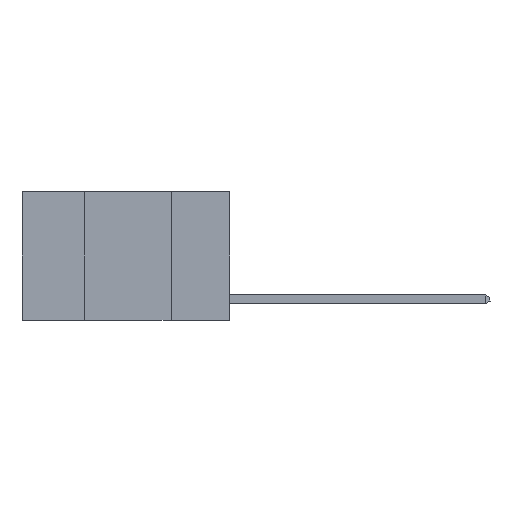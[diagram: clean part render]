
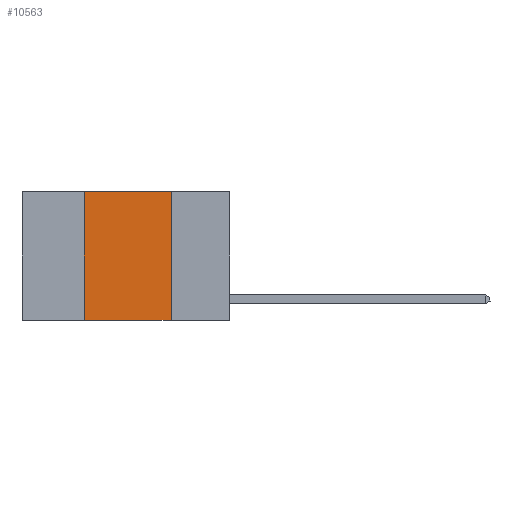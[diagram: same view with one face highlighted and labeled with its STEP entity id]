
A CAD part, left-side view. The second image highlights one B-rep face of the part: STEP entity #10563.
In plain terms, the highlighted planar face has unit normal (-1, 0, 0).
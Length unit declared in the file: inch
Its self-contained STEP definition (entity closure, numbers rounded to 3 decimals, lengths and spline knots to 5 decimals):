
#159 = ORIENTED_EDGE ( 'NONE', *, *, #10945, .T. ) ;
#647 = EDGE_CURVE ( 'NONE', #4507, #5909, #17283, .T. ) ;
#2080 = CARTESIAN_POINT ( 'NONE',  ( 0., 0.42, 0. ) ) ;
#2195 = CARTESIAN_POINT ( 'NONE',  ( 0., 0.6, -0.37 ) ) ;
#2714 = VECTOR ( 'NONE', #12635, 39.37008 ) ;
#2931 = CARTESIAN_POINT ( 'NONE',  ( 0., 0.42, 0. ) ) ;
#3267 = LINE ( 'NONE', #2195, #2714 ) ;
#3363 = CARTESIAN_POINT ( 'NONE',  ( 0., 0.42, -0.37 ) ) ;
#3671 = ORIENTED_EDGE ( 'NONE', *, *, #13306, .F. ) ;
#3960 = CARTESIAN_POINT ( 'NONE',  ( 0., 0.17, 0. ) ) ;
#4500 = VECTOR ( 'NONE', #12670, 39.37008 ) ;
#4507 = VERTEX_POINT ( 'NONE', #2931 ) ;
#5380 = VECTOR ( 'NONE', #19575, 39.37008 ) ;
#5909 = VERTEX_POINT ( 'NONE', #13695 ) ;
#7539 = CARTESIAN_POINT ( 'NONE',  ( 0., 0.6, 0. ) ) ;
#7980 = VECTOR ( 'NONE', #16183, 39.37008 ) ;
#9848 = CARTESIAN_POINT ( 'NONE',  ( 0., 0.6, 0. ) ) ;
#9978 = LINE ( 'NONE', #2080, #5380 ) ;
#10563 = ADVANCED_FACE ( 'NONE', ( #15002 ), #20243, .F. ) ;
#10945 = EDGE_CURVE ( 'NONE', #13084, #15757, #3267, .T. ) ;
#11211 = EDGE_LOOP ( 'NONE', ( #3671, #12945, #17567, #159 ) ) ;
#11629 = DIRECTION ( 'NONE',  ( 0., 0., -1. ) ) ;
#12132 = EDGE_CURVE ( 'NONE', #13084, #4507, #9978, .T. ) ;
#12635 = DIRECTION ( 'NONE',  ( 0., -1., 0. ) ) ;
#12670 = DIRECTION ( 'NONE',  ( 0., 0., -1. ) ) ;
#12945 = ORIENTED_EDGE ( 'NONE', *, *, #647, .F. ) ;
#13084 = VERTEX_POINT ( 'NONE', #3363 ) ;
#13306 = EDGE_CURVE ( 'NONE', #5909, #15757, #18405, .T. ) ;
#13317 = AXIS2_PLACEMENT_3D ( 'NONE', #9848, #22074, #11629 ) ;
#13695 = CARTESIAN_POINT ( 'NONE',  ( 0., 0.17, 0. ) ) ;
#14248 = CARTESIAN_POINT ( 'NONE',  ( 0., 0.17, -0.37 ) ) ;
#15002 = FACE_OUTER_BOUND ( 'NONE', #11211, .T. ) ;
#15757 = VERTEX_POINT ( 'NONE', #14248 ) ;
#16183 = DIRECTION ( 'NONE',  ( 0., -1., 0. ) ) ;
#17283 = LINE ( 'NONE', #7539, #7980 ) ;
#17567 = ORIENTED_EDGE ( 'NONE', *, *, #12132, .F. ) ;
#18405 = LINE ( 'NONE', #3960, #4500 ) ;
#19575 = DIRECTION ( 'NONE',  ( 0., 0., 1. ) ) ;
#20243 = PLANE ( 'NONE',  #13317 ) ;
#22074 = DIRECTION ( 'NONE',  ( 1., 0., 0. ) ) ;
